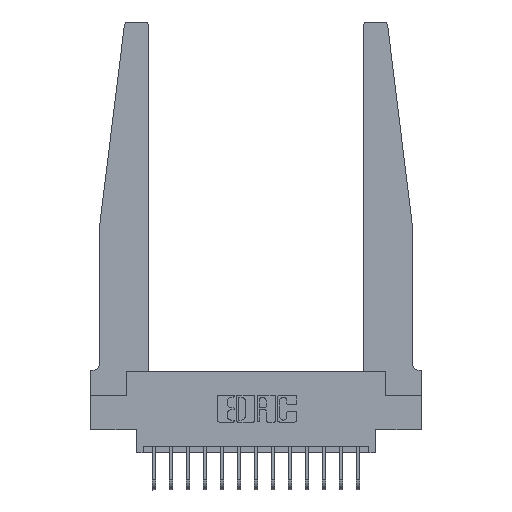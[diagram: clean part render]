
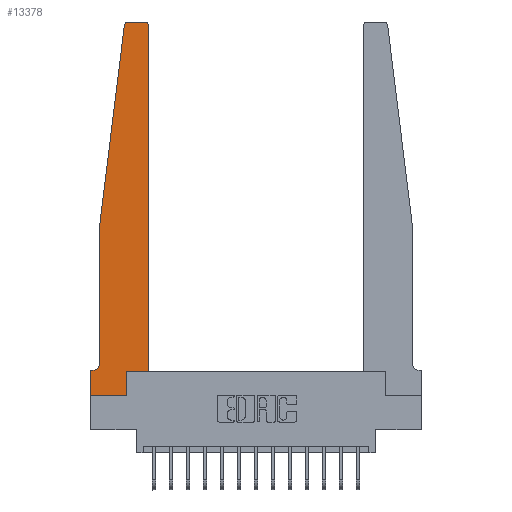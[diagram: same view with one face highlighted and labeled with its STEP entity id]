
A CAD part, top view. The second image highlights one B-rep face of the part: STEP entity #13378.
In plain terms, the highlighted planar face has unit normal (0, 0, 1).
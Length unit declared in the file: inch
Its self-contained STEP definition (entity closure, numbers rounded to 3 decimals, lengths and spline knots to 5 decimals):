
#178 = VERTEX_POINT ( 'NONE', #7150 ) ;
#574 = CARTESIAN_POINT ( 'NONE',  ( 0.2605, 0., 0.37 ) ) ;
#606 = LINE ( 'NONE', #14213, #5295 ) ;
#777 = VERTEX_POINT ( 'NONE', #16302 ) ;
#1155 = EDGE_CURVE ( 'NONE', #14505, #3129, #8971, .T. ) ;
#1158 = DIRECTION ( 'NONE',  ( 1., 0., 0. ) ) ;
#1205 = LINE ( 'NONE', #10294, #3625 ) ;
#1369 = EDGE_CURVE ( 'NONE', #8462, #777, #4717, .T. ) ;
#1761 = DIRECTION ( 'NONE',  ( 0., -1., 0. ) ) ;
#1930 = EDGE_CURVE ( 'NONE', #13176, #18740, #1205, .T. ) ;
#2070 = DIRECTION ( 'NONE',  ( 1., 0., 0. ) ) ;
#2463 = CARTESIAN_POINT ( 'NONE',  ( 0.425, 2.72, 0.37 ) ) ;
#2502 = DIRECTION ( 'NONE',  ( 0., -1., 0. ) ) ;
#2532 = EDGE_CURVE ( 'NONE', #18740, #14505, #12212, .T. ) ;
#3040 = DIRECTION ( 'NONE',  ( -1., 0., 0. ) ) ;
#3097 = DIRECTION ( 'NONE',  ( -1., 0., 0. ) ) ;
#3129 = VERTEX_POINT ( 'NONE', #17446 ) ;
#3619 = DIRECTION ( 'NONE',  ( -1., 0., 0. ) ) ;
#3625 = VECTOR ( 'NONE', #2502, 39.37008 ) ;
#3658 = DIRECTION ( 'NONE',  ( 1., 0., 0. ) ) ;
#3786 = VECTOR ( 'NONE', #19427, 39.37008 ) ;
#4042 = CARTESIAN_POINT ( 'NONE',  ( 0.24675, 2.72367, 0.37 ) ) ;
#4266 = CARTESIAN_POINT ( 'NONE',  ( 0.25, 2.75, 0.37 ) ) ;
#4657 = EDGE_CURVE ( 'NONE', #18715, #9609, #8603, .T. ) ;
#4717 = LINE ( 'NONE', #15275, #17175 ) ;
#4760 = VERTEX_POINT ( 'NONE', #14939 ) ;
#4804 = ORIENTED_EDGE ( 'NONE', *, *, #1930, .T. ) ;
#4855 = EDGE_CURVE ( 'NONE', #178, #4760, #16608, .T. ) ;
#5020 = CARTESIAN_POINT ( 'NONE',  ( 0., 0., 0.37 ) ) ;
#5295 = VECTOR ( 'NONE', #3658, 39.37008 ) ;
#5545 = AXIS2_PLACEMENT_3D ( 'NONE', #6602, #15176, #15360 ) ;
#5586 = EDGE_CURVE ( 'NONE', #9609, #178, #5622, .T. ) ;
#5587 = EDGE_CURVE ( 'NONE', #4760, #15255, #14779, .T. ) ;
#5622 = CIRCLE ( 'NONE', #16989, 0.03 ) ;
#5649 = EDGE_LOOP ( 'NONE', ( #10827, #7751, #13638, #14587, #6719, #9343, #4804, #9695, #11708, #19010, #13981, #12790 ) ) ;
#6592 = EDGE_CURVE ( 'NONE', #777, #18917, #17658, .T. ) ;
#6602 = CARTESIAN_POINT ( 'NONE',  ( 0., 0.1875, 0.37 ) ) ;
#6719 = ORIENTED_EDGE ( 'NONE', *, *, #6592, .T. ) ;
#6721 = EDGE_CURVE ( 'NONE', #15255, #8462, #10343, .T. ) ;
#6739 = CARTESIAN_POINT ( 'NONE',  ( 0., 0., 0.37 ) ) ;
#7150 = CARTESIAN_POINT ( 'NONE',  ( 0.395, 2.75, 0.37 ) ) ;
#7371 = CARTESIAN_POINT ( 'NONE',  ( 0.065, 1.25, 0.37 ) ) ;
#7474 = CARTESIAN_POINT ( 'NONE',  ( 0., 0.1875, 0.37 ) ) ;
#7751 = ORIENTED_EDGE ( 'NONE', *, *, #5587, .T. ) ;
#7758 = DIRECTION ( 'NONE',  ( 0., 0., -1. ) ) ;
#7973 = PLANE ( 'NONE',  #5545 ) ;
#8250 = LINE ( 'NONE', #11496, #18378 ) ;
#8320 = CARTESIAN_POINT ( 'NONE',  ( 0.425, 0.18, 0.37 ) ) ;
#8406 = DIRECTION ( 'NONE',  ( 0., 1., 0. ) ) ;
#8462 = VERTEX_POINT ( 'NONE', #11600 ) ;
#8603 = LINE ( 'NONE', #8320, #13516 ) ;
#8622 = VECTOR ( 'NONE', #15003, 39.37008 ) ;
#8971 = LINE ( 'NONE', #10178, #8622 ) ;
#9343 = ORIENTED_EDGE ( 'NONE', *, *, #18510, .T. ) ;
#9609 = VERTEX_POINT ( 'NONE', #2463 ) ;
#9695 = ORIENTED_EDGE ( 'NONE', *, *, #2532, .T. ) ;
#10178 = CARTESIAN_POINT ( 'NONE',  ( 0.2605, 0.18, 0.37 ) ) ;
#10294 = CARTESIAN_POINT ( 'NONE',  ( 0., 0., 0.37 ) ) ;
#10343 = LINE ( 'NONE', #7371, #3786 ) ;
#10827 = ORIENTED_EDGE ( 'NONE', *, *, #4855, .T. ) ;
#11496 = CARTESIAN_POINT ( 'NONE',  ( 0.065, 0.1875, 0.37 ) ) ;
#11600 = CARTESIAN_POINT ( 'NONE',  ( 0.065, 1.25, 0.37 ) ) ;
#11708 = ORIENTED_EDGE ( 'NONE', *, *, #1155, .T. ) ;
#11722 = DIRECTION ( 'NONE',  ( 0., 0., 1. ) ) ;
#12212 = LINE ( 'NONE', #5020, #14351 ) ;
#12790 = ORIENTED_EDGE ( 'NONE', *, *, #5586, .T. ) ;
#13176 = VERTEX_POINT ( 'NONE', #7474 ) ;
#13375 = CARTESIAN_POINT ( 'NONE',  ( 0.015, 0.2375, 0.37 ) ) ;
#13378 = ADVANCED_FACE ( 'NONE', ( #14078 ), #7973, .T. ) ;
#13516 = VECTOR ( 'NONE', #8406, 39.37008 ) ;
#13638 = ORIENTED_EDGE ( 'NONE', *, *, #6721, .T. ) ;
#13981 = ORIENTED_EDGE ( 'NONE', *, *, #4657, .T. ) ;
#14078 = FACE_OUTER_BOUND ( 'NONE', #5649, .T. ) ;
#14166 = AXIS2_PLACEMENT_3D ( 'NONE', #13375, #7758, #3040 ) ;
#14213 = CARTESIAN_POINT ( 'NONE',  ( 0.425, 0.18, 0.37 ) ) ;
#14351 = VECTOR ( 'NONE', #2070, 39.37008 ) ;
#14505 = VERTEX_POINT ( 'NONE', #574 ) ;
#14587 = ORIENTED_EDGE ( 'NONE', *, *, #1369, .T. ) ;
#14779 = CIRCLE ( 'NONE', #17312, 0.03 ) ;
#14939 = CARTESIAN_POINT ( 'NONE',  ( 0.27653, 2.75, 0.37 ) ) ;
#15003 = DIRECTION ( 'NONE',  ( 0., 1., 0. ) ) ;
#15092 = EDGE_CURVE ( 'NONE', #3129, #18715, #606, .T. ) ;
#15112 = VECTOR ( 'NONE', #3097, 39.37008 ) ;
#15176 = DIRECTION ( 'NONE',  ( 0., 0., 1. ) ) ;
#15255 = VERTEX_POINT ( 'NONE', #4042 ) ;
#15275 = CARTESIAN_POINT ( 'NONE',  ( 0.065, 1.25, 0.37 ) ) ;
#15360 = DIRECTION ( 'NONE',  ( 1., 0., 0. ) ) ;
#16159 = CARTESIAN_POINT ( 'NONE',  ( 0.27653, 2.72, 0.37 ) ) ;
#16302 = CARTESIAN_POINT ( 'NONE',  ( 0.065, 0.2375, 0.37 ) ) ;
#16608 = LINE ( 'NONE', #4266, #15112 ) ;
#16733 = CARTESIAN_POINT ( 'NONE',  ( 0.425, 0.18, 0.37 ) ) ;
#16989 = AXIS2_PLACEMENT_3D ( 'NONE', #19244, #11722, #19431 ) ;
#17175 = VECTOR ( 'NONE', #1761, 39.37008 ) ;
#17312 = AXIS2_PLACEMENT_3D ( 'NONE', #16159, #17853, #1158 ) ;
#17446 = CARTESIAN_POINT ( 'NONE',  ( 0.2605, 0.18, 0.37 ) ) ;
#17658 = CIRCLE ( 'NONE', #14166, 0.05 ) ;
#17853 = DIRECTION ( 'NONE',  ( 0., 0., 1. ) ) ;
#18378 = VECTOR ( 'NONE', #3619, 39.37008 ) ;
#18510 = EDGE_CURVE ( 'NONE', #18917, #13176, #8250, .T. ) ;
#18715 = VERTEX_POINT ( 'NONE', #16733 ) ;
#18740 = VERTEX_POINT ( 'NONE', #6739 ) ;
#18917 = VERTEX_POINT ( 'NONE', #19459 ) ;
#19010 = ORIENTED_EDGE ( 'NONE', *, *, #15092, .T. ) ;
#19244 = CARTESIAN_POINT ( 'NONE',  ( 0.395, 2.72, 0.37 ) ) ;
#19427 = DIRECTION ( 'NONE',  ( -0.122, -0.992, 0. ) ) ;
#19431 = DIRECTION ( 'NONE',  ( 1., 0., 0. ) ) ;
#19459 = CARTESIAN_POINT ( 'NONE',  ( 0.015, 0.1875, 0.37 ) ) ;
